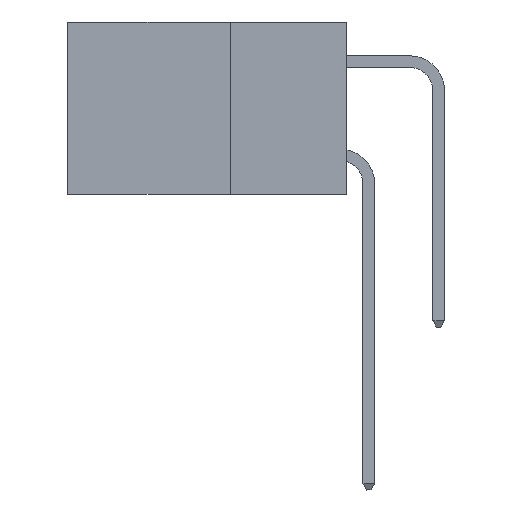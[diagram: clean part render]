
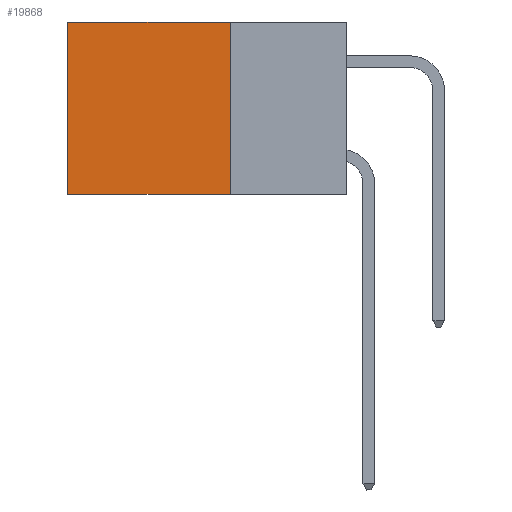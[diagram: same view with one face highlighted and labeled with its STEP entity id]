
A CAD part, left-side view. The second image highlights one B-rep face of the part: STEP entity #19868.
In plain terms, the highlighted planar face has unit normal (-1, 0, 0).
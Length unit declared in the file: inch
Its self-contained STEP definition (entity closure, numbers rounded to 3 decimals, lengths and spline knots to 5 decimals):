
#325 = ORIENTED_EDGE ( 'NONE', *, *, #7566, .F. ) ;
#497 = DIRECTION ( 'NONE',  ( 0., 1., 0. ) ) ;
#506 = VECTOR ( 'NONE', #21059, 39.37008 ) ;
#998 = CARTESIAN_POINT ( 'NONE',  ( 0.2875, 0.6, 0. ) ) ;
#1271 = CARTESIAN_POINT ( 'NONE',  ( 0.2875, 0.6, 0. ) ) ;
#1836 = FACE_OUTER_BOUND ( 'NONE', #4273, .T. ) ;
#1846 = ORIENTED_EDGE ( 'NONE', *, *, #20593, .F. ) ;
#1862 = CARTESIAN_POINT ( 'NONE',  ( 0.2875, 0.25, -0.37 ) ) ;
#2353 = EDGE_CURVE ( 'NONE', #15265, #23076, #21746, .T. ) ;
#3434 = DIRECTION ( 'NONE',  ( 0., 0., -1. ) ) ;
#4273 = EDGE_LOOP ( 'NONE', ( #11662, #1846, #325, #15520 ) ) ;
#7428 = VECTOR ( 'NONE', #23057, 39.37008 ) ;
#7566 = EDGE_CURVE ( 'NONE', #13279, #10289, #13409, .T. ) ;
#9521 = CARTESIAN_POINT ( 'NONE',  ( 0.2875, 0.25, 0. ) ) ;
#10080 = CARTESIAN_POINT ( 'NONE',  ( 0.2875, 0.25, 0. ) ) ;
#10289 = VERTEX_POINT ( 'NONE', #1862 ) ;
#10673 = LINE ( 'NONE', #17138, #14714 ) ;
#10890 = DIRECTION ( 'NONE',  ( 1., 0., 0. ) ) ;
#11662 = ORIENTED_EDGE ( 'NONE', *, *, #2353, .T. ) ;
#11999 = CARTESIAN_POINT ( 'NONE',  ( 0.2875, 0.25, 0. ) ) ;
#13279 = VERTEX_POINT ( 'NONE', #9521 ) ;
#13409 = LINE ( 'NONE', #11999, #506 ) ;
#14606 = PLANE ( 'NONE',  #18766 ) ;
#14714 = VECTOR ( 'NONE', #497, 39.37008 ) ;
#15265 = VERTEX_POINT ( 'NONE', #998 ) ;
#15520 = ORIENTED_EDGE ( 'NONE', *, *, #23961, .T. ) ;
#16227 = DIRECTION ( 'NONE',  ( 0., 0., -1. ) ) ;
#17138 = CARTESIAN_POINT ( 'NONE',  ( 0.2875, 0.25, -0.37 ) ) ;
#18766 = AXIS2_PLACEMENT_3D ( 'NONE', #22001, #10890, #3434 ) ;
#19868 = ADVANCED_FACE ( 'NONE', ( #1836 ), #14606, .F. ) ;
#20593 = EDGE_CURVE ( 'NONE', #10289, #23076, #10673, .T. ) ;
#20618 = CARTESIAN_POINT ( 'NONE',  ( 0.2875, 0.6, -0.37 ) ) ;
#21059 = DIRECTION ( 'NONE',  ( 0., 0., -1. ) ) ;
#21746 = LINE ( 'NONE', #1271, #22038 ) ;
#22001 = CARTESIAN_POINT ( 'NONE',  ( 0.2875, 0.25, 0. ) ) ;
#22038 = VECTOR ( 'NONE', #16227, 39.37008 ) ;
#23057 = DIRECTION ( 'NONE',  ( 0., 1., 0. ) ) ;
#23076 = VERTEX_POINT ( 'NONE', #20618 ) ;
#23103 = LINE ( 'NONE', #10080, #7428 ) ;
#23961 = EDGE_CURVE ( 'NONE', #13279, #15265, #23103, .T. ) ;
